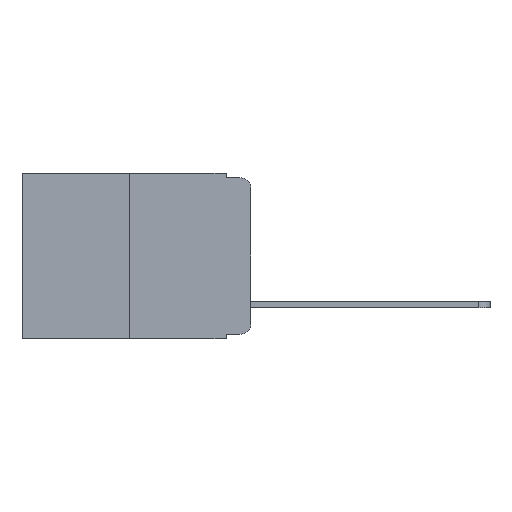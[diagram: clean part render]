
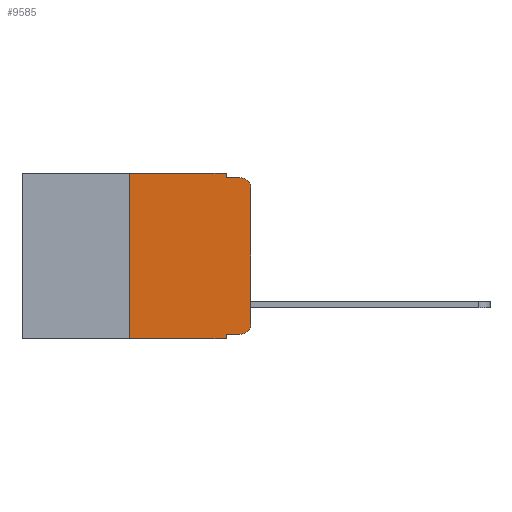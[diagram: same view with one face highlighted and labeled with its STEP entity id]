
A CAD part, left-side view. The second image highlights one B-rep face of the part: STEP entity #9585.
In plain terms, the highlighted planar face has unit normal (-1, 0, 0).
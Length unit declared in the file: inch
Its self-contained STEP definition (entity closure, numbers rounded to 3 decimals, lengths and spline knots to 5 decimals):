
#46 = CARTESIAN_POINT ( 'NONE',  ( 0., 0.25, 0. ) ) ;
#232 = DIRECTION ( 'NONE',  ( 0., 0., -1. ) ) ;
#368 = CIRCLE ( 'NONE', #14775, 0.02 ) ;
#410 = ORIENTED_EDGE ( 'NONE', *, *, #16749, .F. ) ;
#418 = LINE ( 'NONE', #13321, #18543 ) ;
#429 = VERTEX_POINT ( 'NONE', #19048 ) ;
#1288 = CARTESIAN_POINT ( 'NONE',  ( 0., 0.051, 0. ) ) ;
#1640 = DIRECTION ( 'NONE',  ( 0., 0., -1. ) ) ;
#2341 = EDGE_LOOP ( 'NONE', ( #11343, #18844, #4305, #13831, #21703, #410, #14233, #5205, #12346, #11850 ) ) ;
#2363 = CARTESIAN_POINT ( 'NONE',  ( 0., 0.051, -0.333 ) ) ;
#2459 = AXIS2_PLACEMENT_3D ( 'NONE', #18435, #3784, #232 ) ;
#3237 = CARTESIAN_POINT ( 'NONE',  ( 0., 0.051, 0. ) ) ;
#3784 = DIRECTION ( 'NONE',  ( -1., 0., 0. ) ) ;
#3807 = CARTESIAN_POINT ( 'NONE',  ( 0., 0.051, -0.343 ) ) ;
#4276 = DIRECTION ( 'NONE',  ( 0., -1., 0. ) ) ;
#4305 = ORIENTED_EDGE ( 'NONE', *, *, #21842, .F. ) ;
#4408 = CARTESIAN_POINT ( 'NONE',  ( 0., 0.051, -0.01 ) ) ;
#4498 = VECTOR ( 'NONE', #10509, 39.37008 ) ;
#4787 = LINE ( 'NONE', #15688, #4498 ) ;
#5205 = ORIENTED_EDGE ( 'NONE', *, *, #20659, .F. ) ;
#5674 = CARTESIAN_POINT ( 'NONE',  ( 0., 0.051, 0. ) ) ;
#5942 = CARTESIAN_POINT ( 'NONE',  ( 0., 0.051, -0.333 ) ) ;
#6864 = VERTEX_POINT ( 'NONE', #7822 ) ;
#7822 = CARTESIAN_POINT ( 'NONE',  ( 0., 0., -0.03 ) ) ;
#7862 = DIRECTION ( 'NONE',  ( 0., 0., 1. ) ) ;
#8036 = DIRECTION ( 'NONE',  ( 0., 0., -1. ) ) ;
#8785 = VERTEX_POINT ( 'NONE', #46 ) ;
#8913 = CARTESIAN_POINT ( 'NONE',  ( 0., 0.473, 0. ) ) ;
#9065 = EDGE_CURVE ( 'NONE', #6864, #429, #368, .T. ) ;
#9194 = VECTOR ( 'NONE', #23358, 39.37008 ) ;
#9531 = VECTOR ( 'NONE', #17526, 39.37008 ) ;
#9585 = ADVANCED_FACE ( 'NONE', ( #11073 ), #9639, .F. ) ;
#9598 = VECTOR ( 'NONE', #1640, 39.37008 ) ;
#9639 = PLANE ( 'NONE',  #10238 ) ;
#9801 = DIRECTION ( 'NONE',  ( 1., 0., 0. ) ) ;
#10116 = DIRECTION ( 'NONE',  ( 0., 0., -1. ) ) ;
#10238 = AXIS2_PLACEMENT_3D ( 'NONE', #11470, #9801, #10116 ) ;
#10509 = DIRECTION ( 'NONE',  ( 0., -1., 0. ) ) ;
#10700 = LINE ( 'NONE', #8913, #20090 ) ;
#10923 = LINE ( 'NONE', #2363, #12369 ) ;
#11073 = FACE_OUTER_BOUND ( 'NONE', #2341, .T. ) ;
#11106 = CARTESIAN_POINT ( 'NONE',  ( 0., 0.02, -0.333 ) ) ;
#11343 = ORIENTED_EDGE ( 'NONE', *, *, #18194, .T. ) ;
#11470 = CARTESIAN_POINT ( 'NONE',  ( 0., 0.473, 0. ) ) ;
#11828 = CARTESIAN_POINT ( 'NONE',  ( 0., 0.473, -0.343 ) ) ;
#11850 = ORIENTED_EDGE ( 'NONE', *, *, #14721, .T. ) ;
#12072 = EDGE_CURVE ( 'NONE', #18679, #14975, #23264, .T. ) ;
#12346 = ORIENTED_EDGE ( 'NONE', *, *, #16410, .T. ) ;
#12369 = VECTOR ( 'NONE', #4276, 39.37008 ) ;
#12517 = VERTEX_POINT ( 'NONE', #4408 ) ;
#13321 = CARTESIAN_POINT ( 'NONE',  ( 0., 0., 0. ) ) ;
#13831 = ORIENTED_EDGE ( 'NONE', *, *, #21867, .F. ) ;
#14118 = VECTOR ( 'NONE', #22482, 39.37008 ) ;
#14215 = VERTEX_POINT ( 'NONE', #16802 ) ;
#14233 = ORIENTED_EDGE ( 'NONE', *, *, #12072, .T. ) ;
#14597 = LINE ( 'NONE', #18160, #9194 ) ;
#14721 = EDGE_CURVE ( 'NONE', #15529, #14215, #15294, .T. ) ;
#14775 = AXIS2_PLACEMENT_3D ( 'NONE', #22478, #18896, #8036 ) ;
#14975 = VERTEX_POINT ( 'NONE', #3807 ) ;
#15294 = CIRCLE ( 'NONE', #2459, 0.02 ) ;
#15397 = EDGE_CURVE ( 'NONE', #8785, #20937, #10700, .T. ) ;
#15529 = VERTEX_POINT ( 'NONE', #11106 ) ;
#15688 = CARTESIAN_POINT ( 'NONE',  ( 0., 0.051, -0.01 ) ) ;
#16373 = LINE ( 'NONE', #1288, #9531 ) ;
#16410 = EDGE_CURVE ( 'NONE', #16966, #15529, #10923, .T. ) ;
#16749 = EDGE_CURVE ( 'NONE', #18679, #8785, #14597, .T. ) ;
#16802 = CARTESIAN_POINT ( 'NONE',  ( 0., 0., -0.313 ) ) ;
#16966 = VERTEX_POINT ( 'NONE', #5942 ) ;
#17526 = DIRECTION ( 'NONE',  ( 0., 0., -1. ) ) ;
#18160 = CARTESIAN_POINT ( 'NONE',  ( 0., 0.25, 0. ) ) ;
#18194 = EDGE_CURVE ( 'NONE', #14215, #6864, #418, .T. ) ;
#18344 = DIRECTION ( 'NONE',  ( 0., -1., 0. ) ) ;
#18435 = CARTESIAN_POINT ( 'NONE',  ( 0., 0.02, -0.313 ) ) ;
#18543 = VECTOR ( 'NONE', #7862, 39.37008 ) ;
#18679 = VERTEX_POINT ( 'NONE', #20535 ) ;
#18844 = ORIENTED_EDGE ( 'NONE', *, *, #9065, .T. ) ;
#18896 = DIRECTION ( 'NONE',  ( -1., 0., 0. ) ) ;
#19048 = CARTESIAN_POINT ( 'NONE',  ( 0., 0.02, -0.01 ) ) ;
#19309 = LINE ( 'NONE', #3237, #9598 ) ;
#20090 = VECTOR ( 'NONE', #18344, 39.37008 ) ;
#20535 = CARTESIAN_POINT ( 'NONE',  ( 0., 0.25, -0.343 ) ) ;
#20659 = EDGE_CURVE ( 'NONE', #16966, #14975, #19309, .T. ) ;
#20937 = VERTEX_POINT ( 'NONE', #5674 ) ;
#21703 = ORIENTED_EDGE ( 'NONE', *, *, #15397, .F. ) ;
#21842 = EDGE_CURVE ( 'NONE', #12517, #429, #4787, .T. ) ;
#21867 = EDGE_CURVE ( 'NONE', #20937, #12517, #16373, .T. ) ;
#22478 = CARTESIAN_POINT ( 'NONE',  ( 0., 0.02, -0.03 ) ) ;
#22482 = DIRECTION ( 'NONE',  ( 0., -1., 0. ) ) ;
#23264 = LINE ( 'NONE', #11828, #14118 ) ;
#23358 = DIRECTION ( 'NONE',  ( 0., 0., 1. ) ) ;
